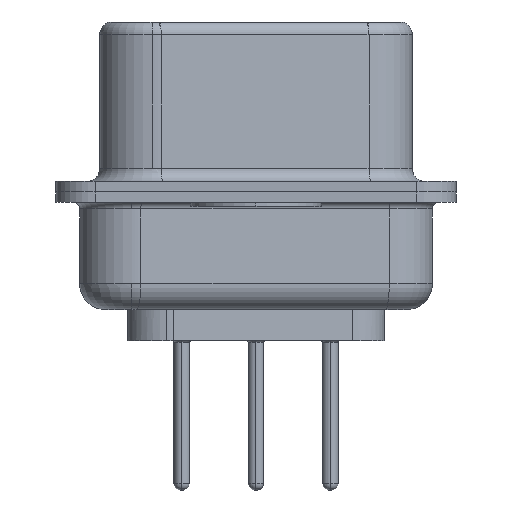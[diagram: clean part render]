
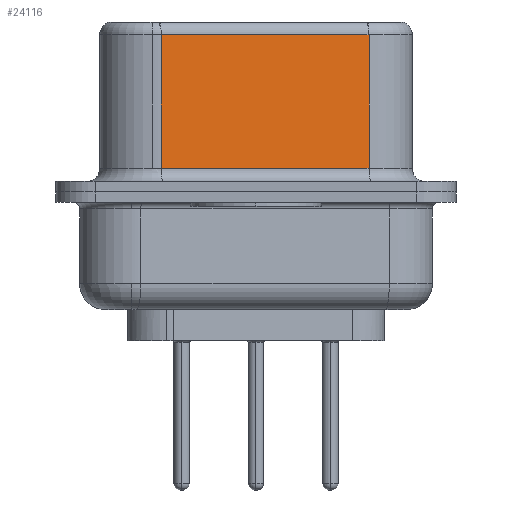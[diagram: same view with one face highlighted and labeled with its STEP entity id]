
A CAD part, left-side view. The second image highlights one B-rep face of the part: STEP entity #24116.
In plain terms, the highlighted planar face has unit normal (-0.985, -0.174, 0).
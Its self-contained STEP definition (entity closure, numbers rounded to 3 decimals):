
#581 = FACE_OUTER_BOUND ( 'NONE', #10058, .T. ) ;
#1399 = LINE ( 'NONE', #20852, #20103 ) ;
#2395 = PLANE ( 'NONE',  #21792 ) ;
#2537 = CARTESIAN_POINT ( 'NONE',  ( 3.73, 3.628, 0.9 ) ) ;
#3644 = DIRECTION ( 'NONE',  ( 0., 0., -1. ) ) ;
#4813 = CARTESIAN_POINT ( 'NONE',  ( 5.132, -4.322, 6.02 ) ) ;
#6468 = ORIENTED_EDGE ( 'NONE', *, *, #15804, .T. ) ;
#6576 = DIRECTION ( 'NONE',  ( 0.985, 0.174, 0. ) ) ;
#7417 = ORIENTED_EDGE ( 'NONE', *, *, #21625, .T. ) ;
#7964 = CARTESIAN_POINT ( 'NONE',  ( 5.132, -4.322, 6.52 ) ) ;
#8289 = EDGE_CURVE ( 'NONE', #27082, #24529, #26593, .T. ) ;
#9077 = DIRECTION ( 'NONE',  ( -0.174, 0.985, 0. ) ) ;
#9382 = VERTEX_POINT ( 'NONE', #2537 ) ;
#10058 = EDGE_LOOP ( 'NONE', ( #18461, #7417, #14217, #6468 ) ) ;
#10785 = DIRECTION ( 'NONE',  ( 0., 0., -1. ) ) ;
#10882 = CARTESIAN_POINT ( 'NONE',  ( 5.132, -4.322, 6.52 ) ) ;
#11723 = VECTOR ( 'NONE', #10785, 1000. ) ;
#12046 = EDGE_CURVE ( 'NONE', #24787, #9382, #22764, .T. ) ;
#12065 = CARTESIAN_POINT ( 'NONE',  ( 5.132, -4.322, 6.02 ) ) ;
#14217 = ORIENTED_EDGE ( 'NONE', *, *, #12046, .T. ) ;
#15684 = CARTESIAN_POINT ( 'NONE',  ( 5.132, -4.322, 0.9 ) ) ;
#15804 = EDGE_CURVE ( 'NONE', #9382, #24529, #1399, .T. ) ;
#18161 = VECTOR ( 'NONE', #3644, 1000. ) ;
#18461 = ORIENTED_EDGE ( 'NONE', *, *, #8289, .F. ) ;
#18909 = DIRECTION ( 'NONE',  ( 0.174, -0.985, 0. ) ) ;
#18980 = CARTESIAN_POINT ( 'NONE',  ( 3.73, 3.628, 6.02 ) ) ;
#20103 = VECTOR ( 'NONE', #18909, 1000. ) ;
#20551 = LINE ( 'NONE', #12065, #21196 ) ;
#20852 = CARTESIAN_POINT ( 'NONE',  ( 5.132, -4.322, 0.9 ) ) ;
#21196 = VECTOR ( 'NONE', #22912, 1000. ) ;
#21625 = EDGE_CURVE ( 'NONE', #27082, #24787, #20551, .T. ) ;
#21792 = AXIS2_PLACEMENT_3D ( 'NONE', #10882, #6576, #9077 ) ;
#22764 = LINE ( 'NONE', #25527, #11723 ) ;
#22912 = DIRECTION ( 'NONE',  ( -0.174, 0.985, 0. ) ) ;
#24116 = ADVANCED_FACE ( 'NONE', ( #581 ), #2395, .F. ) ;
#24529 = VERTEX_POINT ( 'NONE', #15684 ) ;
#24787 = VERTEX_POINT ( 'NONE', #18980 ) ;
#25527 = CARTESIAN_POINT ( 'NONE',  ( 3.73, 3.628, 6.52 ) ) ;
#26593 = LINE ( 'NONE', #7964, #18161 ) ;
#27082 = VERTEX_POINT ( 'NONE', #4813 ) ;
